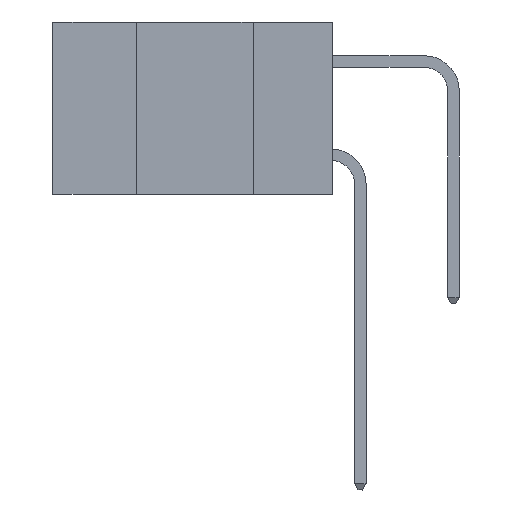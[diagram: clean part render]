
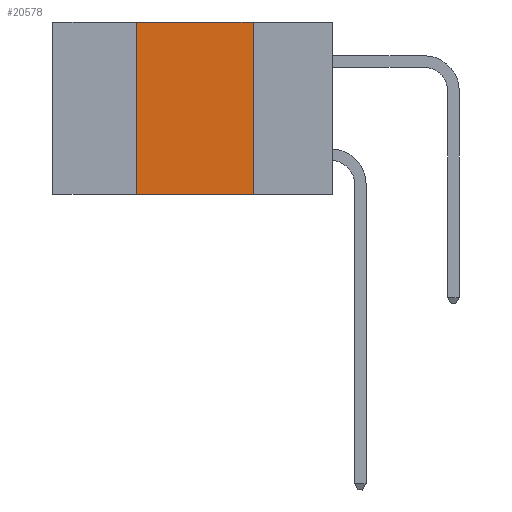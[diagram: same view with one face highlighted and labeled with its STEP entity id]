
A CAD part, left-side view. The second image highlights one B-rep face of the part: STEP entity #20578.
In plain terms, the highlighted planar face has unit normal (-1, 0, 0).
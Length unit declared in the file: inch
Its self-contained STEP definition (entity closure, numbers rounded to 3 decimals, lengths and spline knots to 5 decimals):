
#427 = CARTESIAN_POINT ( 'NONE',  ( 0., 0.42, -0.37 ) ) ;
#1116 = LINE ( 'NONE', #18986, #25283 ) ;
#1863 = FACE_OUTER_BOUND ( 'NONE', #15749, .T. ) ;
#3593 = CARTESIAN_POINT ( 'NONE',  ( 0., 0.6, -0.37 ) ) ;
#4208 = DIRECTION ( 'NONE',  ( 0., 0., -1. ) ) ;
#4601 = VERTEX_POINT ( 'NONE', #12935 ) ;
#4622 = EDGE_CURVE ( 'NONE', #23627, #4601, #14508, .T. ) ;
#5736 = CARTESIAN_POINT ( 'NONE',  ( 0., 0.6, 0. ) ) ;
#5857 = EDGE_CURVE ( 'NONE', #11397, #13011, #1116, .T. ) ;
#6195 = ORIENTED_EDGE ( 'NONE', *, *, #8931, .F. ) ;
#7955 = EDGE_CURVE ( 'NONE', #23627, #13011, #33996, .T. ) ;
#8931 = EDGE_CURVE ( 'NONE', #4601, #11397, #21017, .T. ) ;
#9904 = CARTESIAN_POINT ( 'NONE',  ( 0., 0.42, 0. ) ) ;
#10915 = CARTESIAN_POINT ( 'NONE',  ( 0., 0.17, 0. ) ) ;
#11073 = DIRECTION ( 'NONE',  ( 0., 0., -1. ) ) ;
#11397 = VERTEX_POINT ( 'NONE', #10915 ) ;
#12368 = CARTESIAN_POINT ( 'NONE',  ( 0., 0.6, 0. ) ) ;
#12935 = CARTESIAN_POINT ( 'NONE',  ( 0., 0.42, 0. ) ) ;
#13011 = VERTEX_POINT ( 'NONE', #13145 ) ;
#13145 = CARTESIAN_POINT ( 'NONE',  ( 0., 0.17, -0.37 ) ) ;
#14508 = LINE ( 'NONE', #9904, #18282 ) ;
#14705 = PLANE ( 'NONE',  #32953 ) ;
#15547 = ORIENTED_EDGE ( 'NONE', *, *, #5857, .F. ) ;
#15749 = EDGE_LOOP ( 'NONE', ( #15547, #6195, #30307, #19062 ) ) ;
#16959 = VECTOR ( 'NONE', #32822, 39.37008 ) ;
#18282 = VECTOR ( 'NONE', #28170, 39.37008 ) ;
#18986 = CARTESIAN_POINT ( 'NONE',  ( 0., 0.17, 0. ) ) ;
#19062 = ORIENTED_EDGE ( 'NONE', *, *, #7955, .T. ) ;
#20578 = ADVANCED_FACE ( 'NONE', ( #1863 ), #14705, .F. ) ;
#21017 = LINE ( 'NONE', #5736, #27694 ) ;
#23627 = VERTEX_POINT ( 'NONE', #427 ) ;
#25283 = VECTOR ( 'NONE', #11073, 39.37008 ) ;
#27694 = VECTOR ( 'NONE', #32472, 39.37008 ) ;
#28170 = DIRECTION ( 'NONE',  ( 0., 0., 1. ) ) ;
#30307 = ORIENTED_EDGE ( 'NONE', *, *, #4622, .F. ) ;
#30959 = DIRECTION ( 'NONE',  ( 1., 0., 0. ) ) ;
#32472 = DIRECTION ( 'NONE',  ( 0., -1., 0. ) ) ;
#32822 = DIRECTION ( 'NONE',  ( 0., -1., 0. ) ) ;
#32953 = AXIS2_PLACEMENT_3D ( 'NONE', #12368, #30959, #4208 ) ;
#33996 = LINE ( 'NONE', #3593, #16959 ) ;
